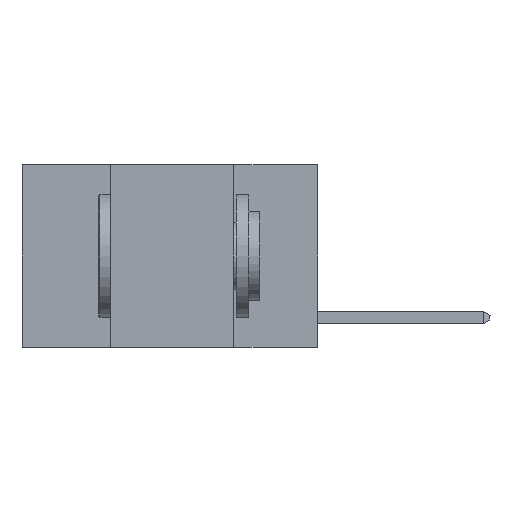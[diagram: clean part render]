
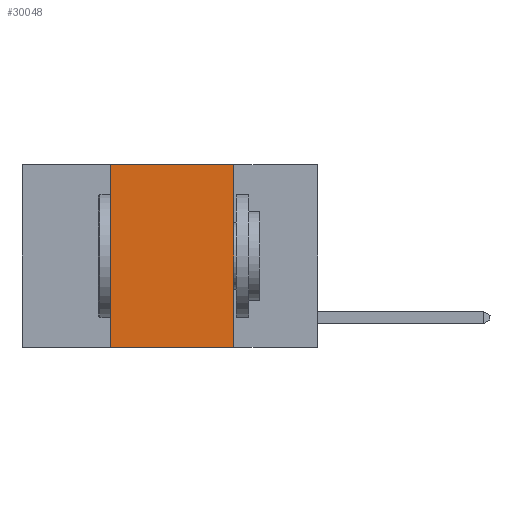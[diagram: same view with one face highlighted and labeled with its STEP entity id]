
A CAD part, left-side view. The second image highlights one B-rep face of the part: STEP entity #30048.
In plain terms, the highlighted planar face has unit normal (-1, 0, 0).
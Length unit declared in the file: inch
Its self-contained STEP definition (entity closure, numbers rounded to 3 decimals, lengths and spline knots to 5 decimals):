
#202 = DIRECTION ( 'NONE',  ( 0., 0., -1. ) ) ;
#1582 = CARTESIAN_POINT ( 'NONE',  ( 0., 0.42, 0. ) ) ;
#3825 = ORIENTED_EDGE ( 'NONE', *, *, #25595, .F. ) ;
#5690 = VECTOR ( 'NONE', #26445, 39.37008 ) ;
#6475 = VERTEX_POINT ( 'NONE', #21908 ) ;
#6661 = CARTESIAN_POINT ( 'NONE',  ( 0., 0.6, -0.37 ) ) ;
#6668 = DIRECTION ( 'NONE',  ( 1., 0., 0. ) ) ;
#6807 = LINE ( 'NONE', #17129, #5690 ) ;
#6928 = EDGE_CURVE ( 'NONE', #17420, #28838, #17387, .T. ) ;
#7141 = EDGE_CURVE ( 'NONE', #6475, #24168, #29271, .T. ) ;
#8069 = AXIS2_PLACEMENT_3D ( 'NONE', #26661, #6668, #22533 ) ;
#8603 = DIRECTION ( 'NONE',  ( 0., -1., 0. ) ) ;
#11748 = CARTESIAN_POINT ( 'NONE',  ( 0., 0.17, 0. ) ) ;
#12269 = FACE_OUTER_BOUND ( 'NONE', #24877, .T. ) ;
#13911 = ORIENTED_EDGE ( 'NONE', *, *, #29900, .T. ) ;
#15106 = VECTOR ( 'NONE', #202, 39.37008 ) ;
#17011 = VECTOR ( 'NONE', #30128, 39.37008 ) ;
#17129 = CARTESIAN_POINT ( 'NONE',  ( 0., 0.6, 0. ) ) ;
#17387 = LINE ( 'NONE', #1582, #17011 ) ;
#17420 = VERTEX_POINT ( 'NONE', #29267 ) ;
#21270 = VECTOR ( 'NONE', #8603, 39.37008 ) ;
#21908 = CARTESIAN_POINT ( 'NONE',  ( 0., 0.17, 0. ) ) ;
#22533 = DIRECTION ( 'NONE',  ( 0., 0., -1. ) ) ;
#22674 = ORIENTED_EDGE ( 'NONE', *, *, #7141, .F. ) ;
#23497 = LINE ( 'NONE', #6661, #21270 ) ;
#23534 = PLANE ( 'NONE',  #8069 ) ;
#23791 = CARTESIAN_POINT ( 'NONE',  ( 0., 0.17, -0.37 ) ) ;
#24168 = VERTEX_POINT ( 'NONE', #23791 ) ;
#24667 = ORIENTED_EDGE ( 'NONE', *, *, #6928, .F. ) ;
#24877 = EDGE_LOOP ( 'NONE', ( #22674, #3825, #24667, #13911 ) ) ;
#25217 = CARTESIAN_POINT ( 'NONE',  ( 0., 0.42, 0. ) ) ;
#25595 = EDGE_CURVE ( 'NONE', #28838, #6475, #6807, .T. ) ;
#26445 = DIRECTION ( 'NONE',  ( 0., -1., 0. ) ) ;
#26661 = CARTESIAN_POINT ( 'NONE',  ( 0., 0.6, 0. ) ) ;
#28838 = VERTEX_POINT ( 'NONE', #25217 ) ;
#29267 = CARTESIAN_POINT ( 'NONE',  ( 0., 0.42, -0.37 ) ) ;
#29271 = LINE ( 'NONE', #11748, #15106 ) ;
#29900 = EDGE_CURVE ( 'NONE', #17420, #24168, #23497, .T. ) ;
#30048 = ADVANCED_FACE ( 'NONE', ( #12269 ), #23534, .F. ) ;
#30128 = DIRECTION ( 'NONE',  ( 0., 0., 1. ) ) ;
